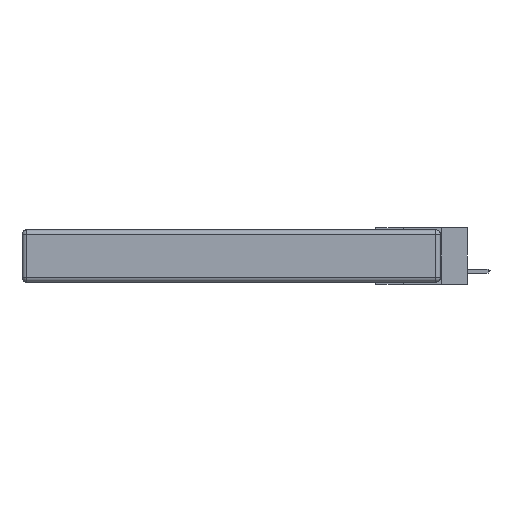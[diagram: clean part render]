
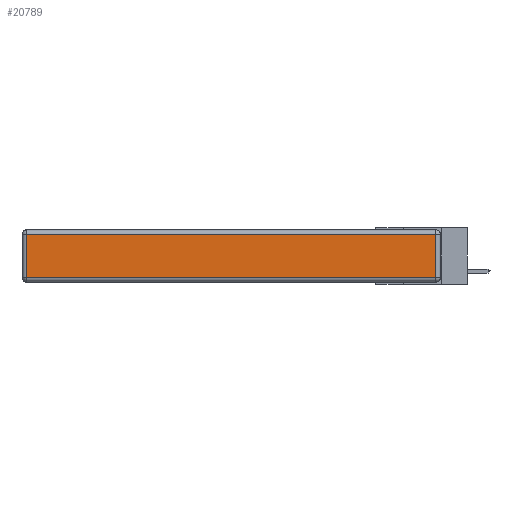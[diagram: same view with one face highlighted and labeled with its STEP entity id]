
A CAD part, left-side view. The second image highlights one B-rep face of the part: STEP entity #20789.
In plain terms, the highlighted planar face has unit normal (-1, 0, 0).
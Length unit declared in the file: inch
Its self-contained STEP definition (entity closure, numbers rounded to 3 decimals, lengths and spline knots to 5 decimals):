
#443 = EDGE_LOOP ( 'NONE', ( #18434, #16704, #18990, #9506 ) ) ;
#468 = EDGE_CURVE ( 'NONE', #10922, #6671, #6794, .T. ) ;
#1774 = VERTEX_POINT ( 'NONE', #6234 ) ;
#3768 = FACE_OUTER_BOUND ( 'NONE', #443, .T. ) ;
#3772 = DIRECTION ( 'NONE',  ( 0., 0., 1. ) ) ;
#3947 = CARTESIAN_POINT ( 'NONE',  ( 0., 0., -0.313 ) ) ;
#6234 = CARTESIAN_POINT ( 'NONE',  ( 0., 0.03, -0.313 ) ) ;
#6671 = VERTEX_POINT ( 'NONE', #7397 ) ;
#6794 = LINE ( 'NONE', #15819, #21749 ) ;
#6875 = CARTESIAN_POINT ( 'NONE',  ( 0., 0.03, -0.343 ) ) ;
#7153 = LINE ( 'NONE', #6875, #21107 ) ;
#7397 = CARTESIAN_POINT ( 'NONE',  ( 0., 2.72, -0.313 ) ) ;
#8826 = DIRECTION ( 'NONE',  ( 0., 0., 1. ) ) ;
#8845 = VERTEX_POINT ( 'NONE', #20165 ) ;
#9506 = ORIENTED_EDGE ( 'NONE', *, *, #468, .T. ) ;
#10922 = VERTEX_POINT ( 'NONE', #25403 ) ;
#11280 = LINE ( 'NONE', #3947, #17262 ) ;
#11513 = CARTESIAN_POINT ( 'NONE',  ( 0., 2.75, -0.03 ) ) ;
#13494 = EDGE_CURVE ( 'NONE', #6671, #1774, #11280, .T. ) ;
#14690 = AXIS2_PLACEMENT_3D ( 'NONE', #18421, #16308, #3772 ) ;
#15065 = EDGE_CURVE ( 'NONE', #8845, #10922, #15169, .T. ) ;
#15169 = LINE ( 'NONE', #11513, #21423 ) ;
#15819 = CARTESIAN_POINT ( 'NONE',  ( 0., 2.72, -0.343 ) ) ;
#16308 = DIRECTION ( 'NONE',  ( -1., 0., 0. ) ) ;
#16485 = PLANE ( 'NONE',  #14690 ) ;
#16704 = ORIENTED_EDGE ( 'NONE', *, *, #23976, .T. ) ;
#17262 = VECTOR ( 'NONE', #18857, 39.37008 ) ;
#18421 = CARTESIAN_POINT ( 'NONE',  ( 0., 0., -0.343 ) ) ;
#18434 = ORIENTED_EDGE ( 'NONE', *, *, #13494, .T. ) ;
#18621 = DIRECTION ( 'NONE',  ( 0., 1., 0. ) ) ;
#18857 = DIRECTION ( 'NONE',  ( 0., -1., 0. ) ) ;
#18990 = ORIENTED_EDGE ( 'NONE', *, *, #15065, .T. ) ;
#20165 = CARTESIAN_POINT ( 'NONE',  ( 0., 0.03, -0.03 ) ) ;
#20789 = ADVANCED_FACE ( 'NONE', ( #3768 ), #16485, .T. ) ;
#21107 = VECTOR ( 'NONE', #8826, 39.37008 ) ;
#21423 = VECTOR ( 'NONE', #18621, 39.37008 ) ;
#21749 = VECTOR ( 'NONE', #22089, 39.37008 ) ;
#22089 = DIRECTION ( 'NONE',  ( 0., 0., -1. ) ) ;
#23976 = EDGE_CURVE ( 'NONE', #1774, #8845, #7153, .T. ) ;
#25403 = CARTESIAN_POINT ( 'NONE',  ( 0., 2.72, -0.03 ) ) ;
